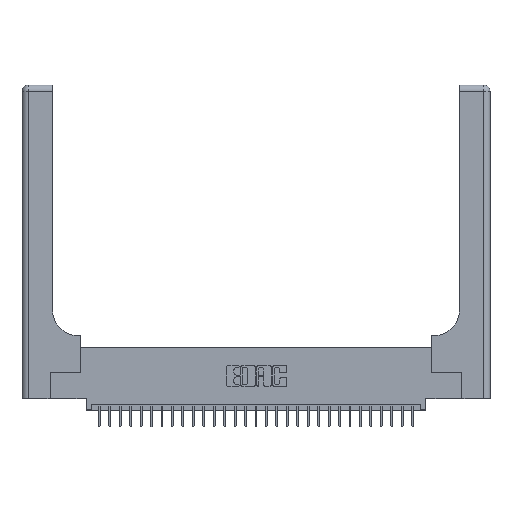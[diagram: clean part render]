
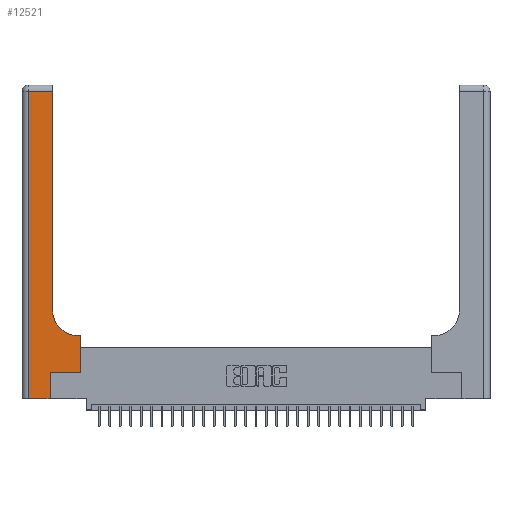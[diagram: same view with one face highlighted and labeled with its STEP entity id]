
A CAD part, top view. The second image highlights one B-rep face of the part: STEP entity #12521.
In plain terms, the highlighted planar face has unit normal (0, 0, 1).
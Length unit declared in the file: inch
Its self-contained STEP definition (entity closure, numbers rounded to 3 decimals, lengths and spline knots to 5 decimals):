
#799 = CARTESIAN_POINT ( 'NONE',  ( 0.5585, 0.25, 0.37 ) ) ;
#1135 = PLANE ( 'NONE',  #3871 ) ;
#1365 = EDGE_CURVE ( 'NONE', #2631, #15837, #1461, .T. ) ;
#1461 = LINE ( 'NONE', #19204, #7199 ) ;
#2261 = DIRECTION ( 'NONE',  ( 1., 0., 0. ) ) ;
#2631 = VERTEX_POINT ( 'NONE', #31216 ) ;
#2705 = CIRCLE ( 'NONE', #25506, 0.25 ) ;
#3619 = DIRECTION ( 'NONE',  ( -1., 0., 0. ) ) ;
#3871 = AXIS2_PLACEMENT_3D ( 'NONE', #18102, #20515, #6021 ) ;
#3890 = EDGE_CURVE ( 'NONE', #6153, #25157, #25983, .T. ) ;
#4096 = ORIENTED_EDGE ( 'NONE', *, *, #8481, .T. ) ;
#4170 = DIRECTION ( 'NONE',  ( -1., 0., 0. ) ) ;
#4679 = EDGE_CURVE ( 'NONE', #15837, #21321, #29659, .T. ) ;
#5043 = ORIENTED_EDGE ( 'NONE', *, *, #20649, .T. ) ;
#5174 = CARTESIAN_POINT ( 'NONE',  ( 0.2915, 0.85, 0.37 ) ) ;
#5488 = LINE ( 'NONE', #26647, #30293 ) ;
#5695 = DIRECTION ( 'NONE',  ( 0., 1., 0. ) ) ;
#5779 = VECTOR ( 'NONE', #11411, 39.37008 ) ;
#6021 = DIRECTION ( 'NONE',  ( -1., 0., 0. ) ) ;
#6153 = VERTEX_POINT ( 'NONE', #10544 ) ;
#7199 = VECTOR ( 'NONE', #2261, 39.37008 ) ;
#7345 = EDGE_CURVE ( 'NONE', #24858, #2631, #5488, .T. ) ;
#8013 = CARTESIAN_POINT ( 'NONE',  ( 0.5585, 0.6, 0.37 ) ) ;
#8463 = VECTOR ( 'NONE', #4170, 39.37008 ) ;
#8481 = EDGE_CURVE ( 'NONE', #25157, #24858, #24997, .T. ) ;
#8544 = CARTESIAN_POINT ( 'NONE',  ( 0.5585, 0.25, 0.37 ) ) ;
#9237 = CARTESIAN_POINT ( 'NONE',  ( 0.5415, 0.6, 0.37 ) ) ;
#9850 = VECTOR ( 'NONE', #5695, 39.37008 ) ;
#10510 = ORIENTED_EDGE ( 'NONE', *, *, #1365, .T. ) ;
#10544 = CARTESIAN_POINT ( 'NONE',  ( 0.06, 2.94, 0.37 ) ) ;
#11411 = DIRECTION ( 'NONE',  ( 1., 0., 0. ) ) ;
#11532 = ORIENTED_EDGE ( 'NONE', *, *, #4679, .T. ) ;
#12146 = VERTEX_POINT ( 'NONE', #18862 ) ;
#12521 = ADVANCED_FACE ( 'NONE', ( #13147 ), #1135, .F. ) ;
#13147 = FACE_OUTER_BOUND ( 'NONE', #21959, .T. ) ;
#13251 = VECTOR ( 'NONE', #29076, 39.37008 ) ;
#13383 = CARTESIAN_POINT ( 'NONE',  ( 0., 2.94, 0.37 ) ) ;
#13699 = DIRECTION ( 'NONE',  ( 0., 0., -1. ) ) ;
#14935 = LINE ( 'NONE', #18675, #8463 ) ;
#14950 = DIRECTION ( 'NONE',  ( 0., 1., 0. ) ) ;
#15837 = VERTEX_POINT ( 'NONE', #8544 ) ;
#17033 = LINE ( 'NONE', #29657, #9850 ) ;
#17318 = CARTESIAN_POINT ( 'NONE',  ( 0.06, 0., 0.37 ) ) ;
#17651 = EDGE_CURVE ( 'NONE', #21321, #27708, #14935, .T. ) ;
#18102 = CARTESIAN_POINT ( 'NONE',  ( 0., 3., 0.37 ) ) ;
#18675 = CARTESIAN_POINT ( 'NONE',  ( 0.2915, 0.6, 0.37 ) ) ;
#18862 = CARTESIAN_POINT ( 'NONE',  ( 0.2915, 2.94, 0.37 ) ) ;
#19204 = CARTESIAN_POINT ( 'NONE',  ( 0.269, 0.25, 0.37 ) ) ;
#19339 = ORIENTED_EDGE ( 'NONE', *, *, #17651, .T. ) ;
#19418 = CARTESIAN_POINT ( 'NONE',  ( 0.06, 3., 0.37 ) ) ;
#19722 = ORIENTED_EDGE ( 'NONE', *, *, #29317, .T. ) ;
#20515 = DIRECTION ( 'NONE',  ( 0., 0., -1. ) ) ;
#20649 = EDGE_CURVE ( 'NONE', #24510, #12146, #17033, .T. ) ;
#20651 = VECTOR ( 'NONE', #3619, 39.37008 ) ;
#21321 = VERTEX_POINT ( 'NONE', #8013 ) ;
#21715 = ORIENTED_EDGE ( 'NONE', *, *, #27456, .T. ) ;
#21959 = EDGE_LOOP ( 'NONE', ( #5043, #21715, #26716, #4096, #27722, #10510, #11532, #19339, #19722 ) ) ;
#22599 = DIRECTION ( 'NONE',  ( 0., 1., 0. ) ) ;
#23332 = VECTOR ( 'NONE', #22599, 39.37008 ) ;
#23389 = CARTESIAN_POINT ( 'NONE',  ( 0., 0., 0.37 ) ) ;
#24510 = VERTEX_POINT ( 'NONE', #5174 ) ;
#24858 = VERTEX_POINT ( 'NONE', #30577 ) ;
#24997 = LINE ( 'NONE', #23389, #5779 ) ;
#25157 = VERTEX_POINT ( 'NONE', #17318 ) ;
#25506 = AXIS2_PLACEMENT_3D ( 'NONE', #28021, #13699, #30413 ) ;
#25983 = LINE ( 'NONE', #19418, #13251 ) ;
#26647 = CARTESIAN_POINT ( 'NONE',  ( 0.269, 0., 0.37 ) ) ;
#26716 = ORIENTED_EDGE ( 'NONE', *, *, #3890, .T. ) ;
#27456 = EDGE_CURVE ( 'NONE', #12146, #6153, #27728, .T. ) ;
#27708 = VERTEX_POINT ( 'NONE', #9237 ) ;
#27722 = ORIENTED_EDGE ( 'NONE', *, *, #7345, .T. ) ;
#27728 = LINE ( 'NONE', #13383, #20651 ) ;
#28021 = CARTESIAN_POINT ( 'NONE',  ( 0.5415, 0.85, 0.37 ) ) ;
#29076 = DIRECTION ( 'NONE',  ( 0., -1., 0. ) ) ;
#29317 = EDGE_CURVE ( 'NONE', #27708, #24510, #2705, .T. ) ;
#29657 = CARTESIAN_POINT ( 'NONE',  ( 0.2915, 3., 0.37 ) ) ;
#29659 = LINE ( 'NONE', #799, #23332 ) ;
#30293 = VECTOR ( 'NONE', #14950, 39.37008 ) ;
#30413 = DIRECTION ( 'NONE',  ( 1., 0., 0. ) ) ;
#30577 = CARTESIAN_POINT ( 'NONE',  ( 0.269, 0., 0.37 ) ) ;
#31216 = CARTESIAN_POINT ( 'NONE',  ( 0.269, 0.25, 0.37 ) ) ;
